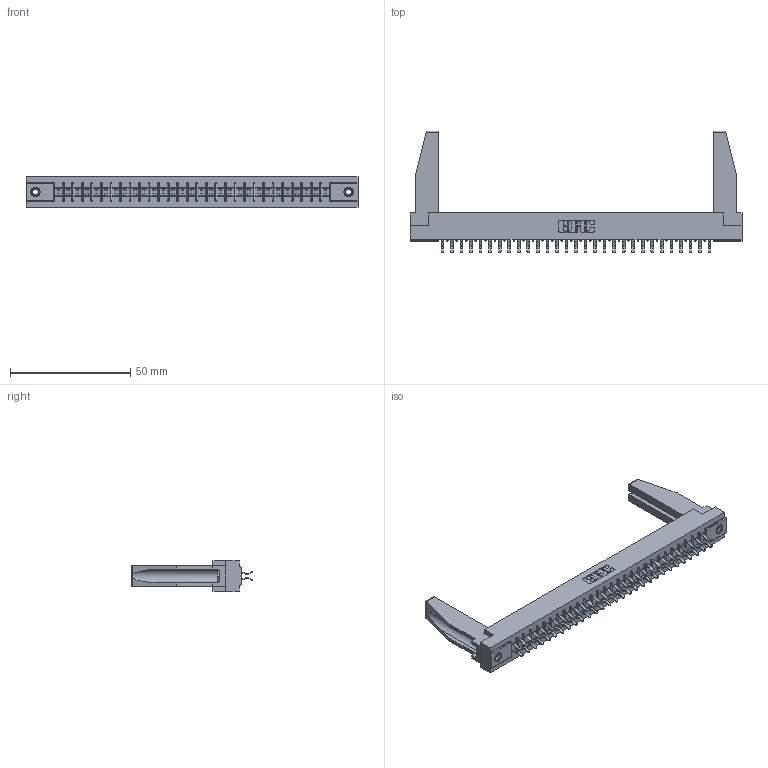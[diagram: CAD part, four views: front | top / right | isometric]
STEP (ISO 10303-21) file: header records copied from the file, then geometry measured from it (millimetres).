
FILE_DESCRIPTION (( 'STEP AP203' ), '1' );
FILE_NAME ('305-058-556-578.STEP', '2019-09-10T00:50:18', ( '' ), ( '' ), 'SwSTEP 2.0', 'SolidWorks 2016', '' );
FILE_SCHEMA (( 'CONFIG_CONTROL_DESIGN' ));
Length unit declared in the file: inch
Products named in the file (5): 345-250-001_345-250-001-102; 305-290-001_556; 305 Part_.156 Dia; 307-220-078; 305-058-556-578
Assembly tree (63 placements, depth 2):
  305-058-556-578
    305 Part_.156 Dia
    305-290-001_556  x58
    345-250-001_345-250-001-102  x2
    307-220-078  x2
Bounding box: 137.92 x 50.67 x 12.7 mm (x, y, z)
Volume: 17893 mm3; surface area: 21876.4 mm2
Topology: 63 solids, 63 shells, 3494 faces, 10013 edges, 6510 vertices
Faces by surface type: plane 1950, cylinder 1412, sphere 116, cone 12, torus 4
Entity records: 35643 total; most frequent: CARTESIAN_POINT 5907, ORIENTED_EDGE 5820, DIRECTION 5686, EDGE_CURVE 2910, LINE 2332, VECTOR 2332, VERTEX_POINT 1856, AXIS2_PLACEMENT_3D 1677
